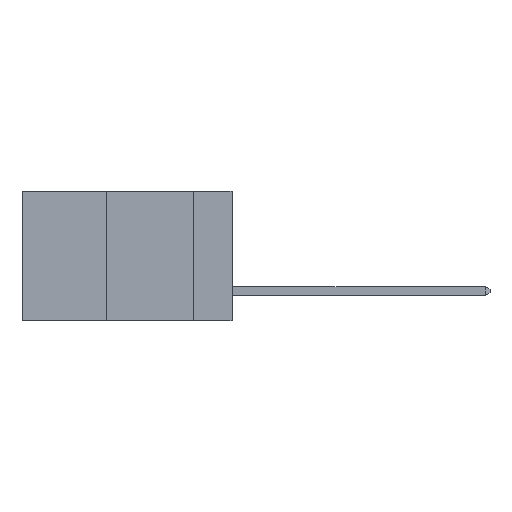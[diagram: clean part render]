
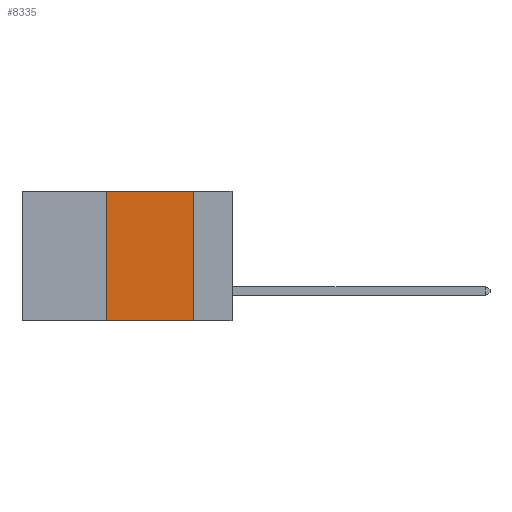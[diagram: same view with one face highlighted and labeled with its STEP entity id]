
A CAD part, left-side view. The second image highlights one B-rep face of the part: STEP entity #8335.
In plain terms, the highlighted planar face has unit normal (-1, 0, 0).
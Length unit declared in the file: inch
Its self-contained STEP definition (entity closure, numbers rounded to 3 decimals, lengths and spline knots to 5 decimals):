
#195 = DIRECTION ( 'NONE',  ( 0., -1., 0. ) ) ;
#292 = DIRECTION ( 'NONE',  ( 0., -1., 0. ) ) ;
#606 = VECTOR ( 'NONE', #13018, 39.37008 ) ;
#827 = VERTEX_POINT ( 'NONE', #4512 ) ;
#1220 = ORIENTED_EDGE ( 'NONE', *, *, #9804, .F. ) ;
#1830 = EDGE_LOOP ( 'NONE', ( #1998, #1220, #14092, #6625 ) ) ;
#1998 = ORIENTED_EDGE ( 'NONE', *, *, #15007, .F. ) ;
#3687 = VERTEX_POINT ( 'NONE', #8001 ) ;
#4512 = CARTESIAN_POINT ( 'NONE',  ( 0., 0.36, 0. ) ) ;
#4781 = VECTOR ( 'NONE', #292, 39.37008 ) ;
#6625 = ORIENTED_EDGE ( 'NONE', *, *, #12342, .T. ) ;
#6736 = CARTESIAN_POINT ( 'NONE',  ( 0., 0.6, 0. ) ) ;
#6906 = DIRECTION ( 'NONE',  ( 1., 0., 0. ) ) ;
#7527 = CARTESIAN_POINT ( 'NONE',  ( 0., 0.36, -0.37 ) ) ;
#8001 = CARTESIAN_POINT ( 'NONE',  ( 0., 0.11, -0.37 ) ) ;
#8269 = FACE_OUTER_BOUND ( 'NONE', #1830, .T. ) ;
#8335 = ADVANCED_FACE ( 'NONE', ( #8269 ), #14582, .F. ) ;
#9194 = EDGE_CURVE ( 'NONE', #14792, #827, #16107, .T. ) ;
#9282 = CARTESIAN_POINT ( 'NONE',  ( 0., 0.36, 0. ) ) ;
#9804 = EDGE_CURVE ( 'NONE', #827, #9807, #13705, .T. ) ;
#9807 = VERTEX_POINT ( 'NONE', #14426 ) ;
#9879 = VECTOR ( 'NONE', #195, 39.37008 ) ;
#11676 = LINE ( 'NONE', #15795, #4781 ) ;
#12016 = CARTESIAN_POINT ( 'NONE',  ( 0., 0.6, 0. ) ) ;
#12342 = EDGE_CURVE ( 'NONE', #14792, #3687, #11676, .T. ) ;
#13018 = DIRECTION ( 'NONE',  ( 0., 0., -1. ) ) ;
#13705 = LINE ( 'NONE', #6736, #9879 ) ;
#14092 = ORIENTED_EDGE ( 'NONE', *, *, #9194, .F. ) ;
#14426 = CARTESIAN_POINT ( 'NONE',  ( 0., 0.11, 0. ) ) ;
#14447 = DIRECTION ( 'NONE',  ( 0., 0., 1. ) ) ;
#14582 = PLANE ( 'NONE',  #16698 ) ;
#14792 = VERTEX_POINT ( 'NONE', #7527 ) ;
#14801 = LINE ( 'NONE', #15538, #606 ) ;
#15007 = EDGE_CURVE ( 'NONE', #9807, #3687, #14801, .T. ) ;
#15538 = CARTESIAN_POINT ( 'NONE',  ( 0., 0.11, 0. ) ) ;
#15723 = VECTOR ( 'NONE', #14447, 39.37008 ) ;
#15795 = CARTESIAN_POINT ( 'NONE',  ( 0., 0.6, -0.37 ) ) ;
#15874 = DIRECTION ( 'NONE',  ( 0., 0., -1. ) ) ;
#16107 = LINE ( 'NONE', #9282, #15723 ) ;
#16698 = AXIS2_PLACEMENT_3D ( 'NONE', #12016, #6906, #15874 ) ;
